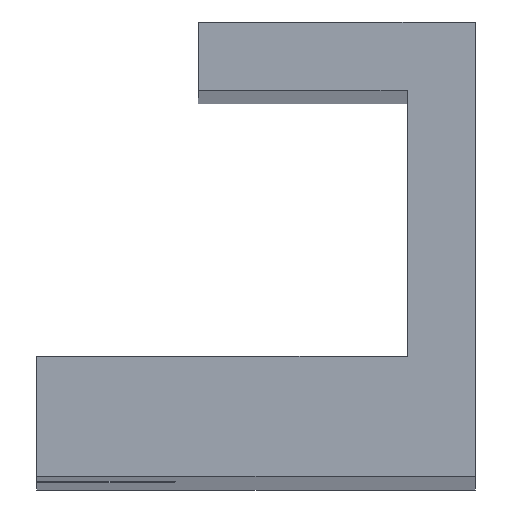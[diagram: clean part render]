
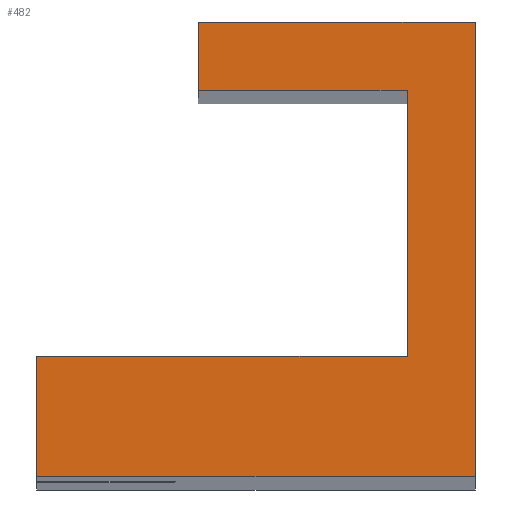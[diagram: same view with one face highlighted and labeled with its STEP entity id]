
A CAD part, top view. The second image highlights one B-rep face of the part: STEP entity #482.
In plain terms, the highlighted planar face has unit normal (0, 0, 1).
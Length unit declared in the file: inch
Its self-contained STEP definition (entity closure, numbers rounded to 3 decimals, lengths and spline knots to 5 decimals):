
#68=FACE_OUTER_BOUND('',#90,.T.);
#90=EDGE_LOOP('',(#351,#352,#353,#354,#355,#356,#357,#358));
#128=LINE('',#717,#172);
#139=LINE('',#738,#183);
#140=LINE('',#742,#184);
#141=LINE('',#744,#185);
#142=LINE('',#745,#186);
#143=LINE('',#747,#187);
#144=LINE('',#749,#188);
#145=LINE('',#750,#189);
#172=VECTOR('',#574,0.3937);
#183=VECTOR('',#593,0.3937);
#184=VECTOR('',#596,0.3937);
#185=VECTOR('',#597,0.3937);
#186=VECTOR('',#598,0.3937);
#187=VECTOR('',#599,0.3937);
#188=VECTOR('',#600,0.3937);
#189=VECTOR('',#601,0.3937);
#216=VERTEX_POINT('',#714);
#217=VERTEX_POINT('',#716);
#223=VERTEX_POINT('',#736);
#224=VERTEX_POINT('',#740);
#225=VERTEX_POINT('',#741);
#226=VERTEX_POINT('',#743);
#227=VERTEX_POINT('',#746);
#228=VERTEX_POINT('',#748);
#264=EDGE_CURVE('',#216,#217,#128,.T.);
#275=EDGE_CURVE('',#223,#216,#139,.T.);
#276=EDGE_CURVE('',#224,#225,#140,.T.);
#277=EDGE_CURVE('',#226,#224,#141,.T.);
#278=EDGE_CURVE('',#217,#226,#142,.T.);
#279=EDGE_CURVE('',#227,#223,#143,.T.);
#280=EDGE_CURVE('',#228,#227,#144,.T.);
#281=EDGE_CURVE('',#225,#228,#145,.T.);
#351=ORIENTED_EDGE('',*,*,#276,.F.);
#352=ORIENTED_EDGE('',*,*,#277,.F.);
#353=ORIENTED_EDGE('',*,*,#278,.F.);
#354=ORIENTED_EDGE('',*,*,#264,.F.);
#355=ORIENTED_EDGE('',*,*,#275,.F.);
#356=ORIENTED_EDGE('',*,*,#279,.F.);
#357=ORIENTED_EDGE('',*,*,#280,.F.);
#358=ORIENTED_EDGE('',*,*,#281,.F.);
#468=PLANE('',#524);
#482=ADVANCED_FACE('',(#68),#468,.F.);
#524=AXIS2_PLACEMENT_3D('',#739,#594,#595);
#574=DIRECTION('',(1.,0.,0.));
#593=DIRECTION('',(0.,1.,0.));
#594=DIRECTION('center_axis',(0.,0.,-1.));
#595=DIRECTION('ref_axis',(-1.,0.,0.));
#596=DIRECTION('',(0.,1.,0.));
#597=DIRECTION('',(-1.,0.,0.));
#598=DIRECTION('',(0.,1.,0.));
#599=DIRECTION('',(-1.,0.,0.));
#600=DIRECTION('',(0.,-1.,0.));
#601=DIRECTION('',(1.,0.,0.));
#714=CARTESIAN_POINT('',(0.,0.10406,6.80194));
#716=CARTESIAN_POINT('',(0.32094,0.10406,6.80194));
#717=CARTESIAN_POINT('',(0.,0.10406,6.80194));
#736=CARTESIAN_POINT('',(0.,0.,6.80194));
#738=CARTESIAN_POINT('',(0.,0.05906,6.80194));
#739=CARTESIAN_POINT('Origin',(0.19,0.19685,6.80194));
#740=CARTESIAN_POINT('',(0.14,0.33465,6.80194));
#741=CARTESIAN_POINT('',(0.14,0.3937,6.80194));
#742=CARTESIAN_POINT('',(0.14,0.26575,6.80194));
#743=CARTESIAN_POINT('',(0.32094,0.33465,6.80194));
#744=CARTESIAN_POINT('',(0.145,0.33465,6.80194));
#745=CARTESIAN_POINT('',(0.32094,0.26575,6.80194));
#746=CARTESIAN_POINT('',(0.38,0.,6.80194));
#747=CARTESIAN_POINT('',(0.095,0.,6.80194));
#748=CARTESIAN_POINT('',(0.38,0.3937,6.80194));
#749=CARTESIAN_POINT('',(0.38,0.09843,6.80194));
#750=CARTESIAN_POINT('',(0.285,0.3937,6.80194));
